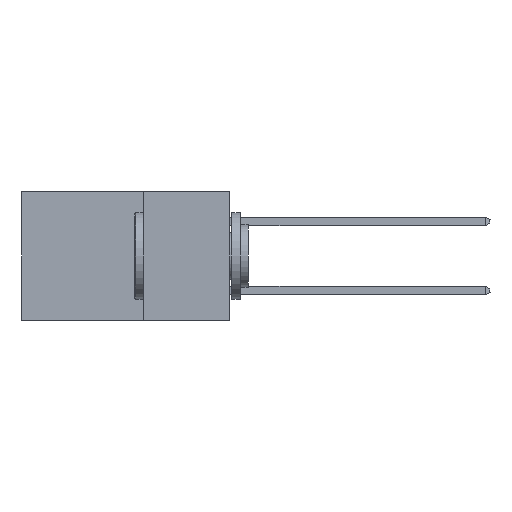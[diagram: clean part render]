
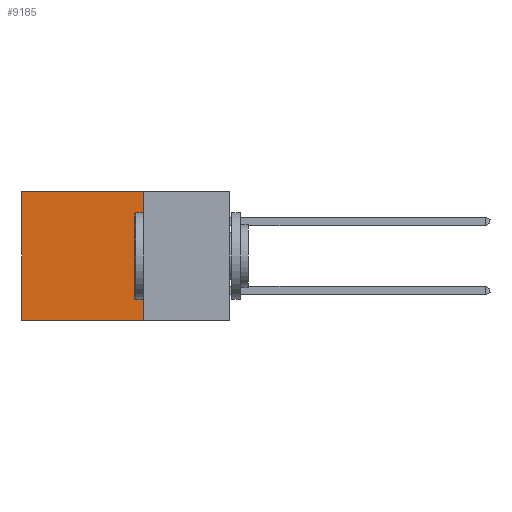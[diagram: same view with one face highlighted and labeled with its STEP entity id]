
A CAD part, left-side view. The second image highlights one B-rep face of the part: STEP entity #9185.
In plain terms, the highlighted planar face has unit normal (-1, 0, 0).
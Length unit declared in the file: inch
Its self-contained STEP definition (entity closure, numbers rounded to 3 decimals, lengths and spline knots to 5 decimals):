
#2242 = ORIENTED_EDGE ( 'NONE', *, *, #7730, .T. ) ;
#2397 = VECTOR ( 'NONE', #12801, 39.37008 ) ;
#2523 = FACE_OUTER_BOUND ( 'NONE', #23132, .T. ) ;
#2706 = EDGE_CURVE ( 'NONE', #4271, #10944, #10192, .T. ) ;
#4271 = VERTEX_POINT ( 'NONE', #16707 ) ;
#6727 = CARTESIAN_POINT ( 'NONE',  ( 0.298, 0.6, 0. ) ) ;
#7730 = EDGE_CURVE ( 'NONE', #4271, #17113, #30834, .T. ) ;
#8609 = VECTOR ( 'NONE', #9097, 39.37008 ) ;
#9097 = DIRECTION ( 'NONE',  ( 0., 0., -1. ) ) ;
#9185 = ADVANCED_FACE ( 'NONE', ( #2523 ), #32198, .F. ) ;
#9320 = VECTOR ( 'NONE', #28208, 39.37008 ) ;
#10192 = LINE ( 'NONE', #24355, #8609 ) ;
#10944 = VERTEX_POINT ( 'NONE', #30634 ) ;
#12801 = DIRECTION ( 'NONE',  ( 0., 1., 0. ) ) ;
#12899 = CARTESIAN_POINT ( 'NONE',  ( 0.298, 0.25, 0. ) ) ;
#13932 = CARTESIAN_POINT ( 'NONE',  ( 0.298, 0.6, -0.37 ) ) ;
#14283 = CARTESIAN_POINT ( 'NONE',  ( 0.298, 0.25, 0. ) ) ;
#15178 = LINE ( 'NONE', #6727, #17137 ) ;
#15577 = ORIENTED_EDGE ( 'NONE', *, *, #27849, .T. ) ;
#16707 = CARTESIAN_POINT ( 'NONE',  ( 0.298, 0.25, 0. ) ) ;
#17113 = VERTEX_POINT ( 'NONE', #23151 ) ;
#17137 = VECTOR ( 'NONE', #27847, 39.37008 ) ;
#20634 = VERTEX_POINT ( 'NONE', #13932 ) ;
#23132 = EDGE_LOOP ( 'NONE', ( #15577, #28078, #26247, #2242 ) ) ;
#23151 = CARTESIAN_POINT ( 'NONE',  ( 0.298, 0.6, 0. ) ) ;
#24355 = CARTESIAN_POINT ( 'NONE',  ( 0.298, 0.25, 0. ) ) ;
#24814 = DIRECTION ( 'NONE',  ( 1., 0., 0. ) ) ;
#25117 = EDGE_CURVE ( 'NONE', #10944, #20634, #30217, .T. ) ;
#26247 = ORIENTED_EDGE ( 'NONE', *, *, #2706, .F. ) ;
#27847 = DIRECTION ( 'NONE',  ( 0., 0., -1. ) ) ;
#27849 = EDGE_CURVE ( 'NONE', #17113, #20634, #15178, .T. ) ;
#27904 = CARTESIAN_POINT ( 'NONE',  ( 0.298, 0.25, -0.37 ) ) ;
#28078 = ORIENTED_EDGE ( 'NONE', *, *, #25117, .F. ) ;
#28208 = DIRECTION ( 'NONE',  ( 0., 1., 0. ) ) ;
#30217 = LINE ( 'NONE', #27904, #2397 ) ;
#30614 = AXIS2_PLACEMENT_3D ( 'NONE', #14283, #24814, #31770 ) ;
#30634 = CARTESIAN_POINT ( 'NONE',  ( 0.298, 0.25, -0.37 ) ) ;
#30834 = LINE ( 'NONE', #12899, #9320 ) ;
#31770 = DIRECTION ( 'NONE',  ( 0., 0., -1. ) ) ;
#32198 = PLANE ( 'NONE',  #30614 ) ;
